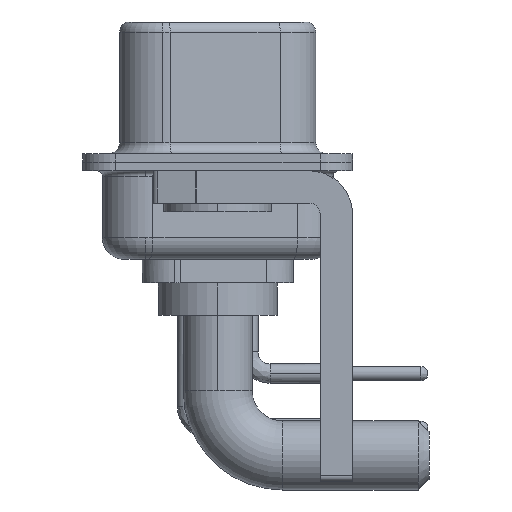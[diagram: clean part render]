
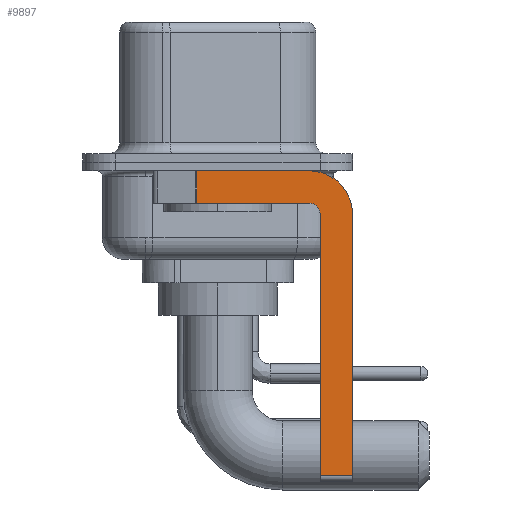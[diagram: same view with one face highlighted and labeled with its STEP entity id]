
A CAD part, left-side view. The second image highlights one B-rep face of the part: STEP entity #9897.
In plain terms, the highlighted planar face has unit normal (-1, 0, 0).
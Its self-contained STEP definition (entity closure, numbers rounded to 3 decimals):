
#367 = PLANE ( 'NONE',  #20569 ) ;
#689 = CARTESIAN_POINT ( 'NONE',  ( -2.9, 0.978, -1.9 ) ) ;
#1030 = LINE ( 'NONE', #17706, #9977 ) ;
#1077 = VERTEX_POINT ( 'NONE', #689 ) ;
#1117 = CARTESIAN_POINT ( 'NONE',  ( -2.9, -4.25, -2.4 ) ) ;
#1243 = EDGE_CURVE ( 'NONE', #19360, #1077, #16159, .T. ) ;
#1424 = VERTEX_POINT ( 'NONE', #6580 ) ;
#2284 = ORIENTED_EDGE ( 'NONE', *, *, #1243, .F. ) ;
#2487 = VERTEX_POINT ( 'NONE', #16591 ) ;
#2780 = LINE ( 'NONE', #12566, #3364 ) ;
#3364 = VECTOR ( 'NONE', #9458, 1000. ) ;
#3404 = DIRECTION ( 'NONE',  ( -1., 0., 0. ) ) ;
#3742 = DIRECTION ( 'NONE',  ( 0., 0., 1. ) ) ;
#3747 = CARTESIAN_POINT ( 'NONE',  ( -2.9, -4.25, -2.4 ) ) ;
#3890 = DIRECTION ( 'NONE',  ( 0., 0., -1. ) ) ;
#4064 = EDGE_CURVE ( 'NONE', #2487, #19360, #4962, .T. ) ;
#4548 = CARTESIAN_POINT ( 'NONE',  ( -2.9, -4.25, -1.9 ) ) ;
#4962 = CIRCLE ( 'NONE', #15115, 0.5 ) ;
#5663 = VERTEX_POINT ( 'NONE', #21495 ) ;
#5921 = EDGE_CURVE ( 'NONE', #13215, #1424, #14132, .T. ) ;
#6148 = CARTESIAN_POINT ( 'NONE',  ( -2.9, -4.25, -1.9 ) ) ;
#6396 = AXIS2_PLACEMENT_3D ( 'NONE', #1117, #9334, #14075 ) ;
#6580 = CARTESIAN_POINT ( 'NONE',  ( -2.9, -6.25, -14.55 ) ) ;
#6722 = VERTEX_POINT ( 'NONE', #11736 ) ;
#6748 = CIRCLE ( 'NONE', #6396, 2. ) ;
#7032 = CARTESIAN_POINT ( 'NONE',  ( -2.9, -4.75, -14.8 ) ) ;
#7209 = ORIENTED_EDGE ( 'NONE', *, *, #18264, .F. ) ;
#7445 = VERTEX_POINT ( 'NONE', #15323 ) ;
#7477 = DIRECTION ( 'NONE',  ( 0., 0., -1. ) ) ;
#8174 = VECTOR ( 'NONE', #12961, 1000. ) ;
#8192 = EDGE_CURVE ( 'NONE', #6722, #2487, #20448, .T. ) ;
#8270 = ORIENTED_EDGE ( 'NONE', *, *, #9693, .F. ) ;
#9334 = DIRECTION ( 'NONE',  ( 1., 0., 0. ) ) ;
#9458 = DIRECTION ( 'NONE',  ( 0., -1., 0. ) ) ;
#9693 = EDGE_CURVE ( 'NONE', #5663, #7445, #2780, .T. ) ;
#9897 = ADVANCED_FACE ( 'NONE', ( #18808 ), #367, .F. ) ;
#9977 = VECTOR ( 'NONE', #7477, 1000. ) ;
#10106 = EDGE_CURVE ( 'NONE', #5663, #1077, #1030, .T. ) ;
#10209 = EDGE_CURVE ( 'NONE', #6722, #1424, #18133, .T. ) ;
#11466 = CARTESIAN_POINT ( 'NONE',  ( -2.9, -6.25, -2.4 ) ) ;
#11643 = CARTESIAN_POINT ( 'NONE',  ( -2.9, -4.25, -14.55 ) ) ;
#11736 = CARTESIAN_POINT ( 'NONE',  ( -2.9, -4.75, -14.55 ) ) ;
#12049 = EDGE_LOOP ( 'NONE', ( #8270, #15031, #2284, #14236, #18894, #18888, #20808, #7209 ) ) ;
#12248 = CARTESIAN_POINT ( 'NONE',  ( -2.9, -6.25, -2.4 ) ) ;
#12566 = CARTESIAN_POINT ( 'NONE',  ( -2.9, 3., -0.4 ) ) ;
#12961 = DIRECTION ( 'NONE',  ( 0., 1., 0. ) ) ;
#13215 = VERTEX_POINT ( 'NONE', #11466 ) ;
#13650 = DIRECTION ( 'NONE',  ( 1., 0., 0. ) ) ;
#14075 = DIRECTION ( 'NONE',  ( 0., 0., -1. ) ) ;
#14132 = LINE ( 'NONE', #12248, #14825 ) ;
#14236 = ORIENTED_EDGE ( 'NONE', *, *, #4064, .F. ) ;
#14825 = VECTOR ( 'NONE', #3890, 1000. ) ;
#15031 = ORIENTED_EDGE ( 'NONE', *, *, #10106, .T. ) ;
#15115 = AXIS2_PLACEMENT_3D ( 'NONE', #15486, #3404, #18787 ) ;
#15170 = DIRECTION ( 'NONE',  ( 0., -1., 0. ) ) ;
#15323 = CARTESIAN_POINT ( 'NONE',  ( -2.9, -4.25, -0.4 ) ) ;
#15486 = CARTESIAN_POINT ( 'NONE',  ( -2.9, -4.25, -2.4 ) ) ;
#15510 = DIRECTION ( 'NONE',  ( 0., 0., -1. ) ) ;
#15577 = VECTOR ( 'NONE', #3742, 1000. ) ;
#16159 = LINE ( 'NONE', #6148, #8174 ) ;
#16591 = CARTESIAN_POINT ( 'NONE',  ( -2.9, -4.75, -2.4 ) ) ;
#17706 = CARTESIAN_POINT ( 'NONE',  ( -2.9, 0.978, -1.9 ) ) ;
#18133 = LINE ( 'NONE', #11643, #21580 ) ;
#18264 = EDGE_CURVE ( 'NONE', #7445, #13215, #6748, .T. ) ;
#18787 = DIRECTION ( 'NONE',  ( 0., 0., 1. ) ) ;
#18808 = FACE_OUTER_BOUND ( 'NONE', #12049, .T. ) ;
#18888 = ORIENTED_EDGE ( 'NONE', *, *, #10209, .T. ) ;
#18894 = ORIENTED_EDGE ( 'NONE', *, *, #8192, .F. ) ;
#19360 = VERTEX_POINT ( 'NONE', #4548 ) ;
#20448 = LINE ( 'NONE', #7032, #15577 ) ;
#20569 = AXIS2_PLACEMENT_3D ( 'NONE', #3747, #13650, #15510 ) ;
#20808 = ORIENTED_EDGE ( 'NONE', *, *, #5921, .F. ) ;
#21495 = CARTESIAN_POINT ( 'NONE',  ( -2.9, 0.978, -0.4 ) ) ;
#21580 = VECTOR ( 'NONE', #15170, 1000. ) ;
